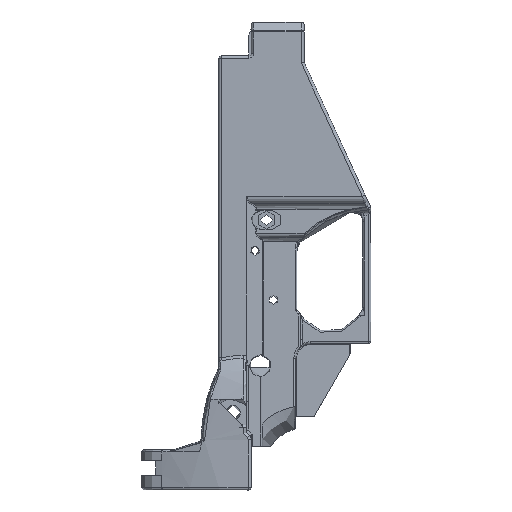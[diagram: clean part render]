
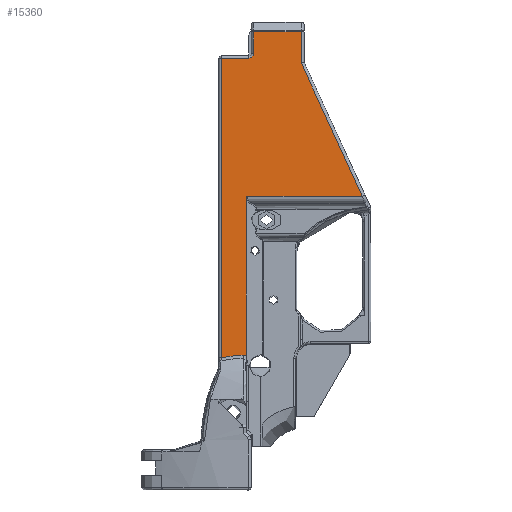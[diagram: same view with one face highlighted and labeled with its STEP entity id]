
A CAD part, left-side view. The second image highlights one B-rep face of the part: STEP entity #15360.
In plain terms, the highlighted planar face has unit normal (-1, 0, 0).
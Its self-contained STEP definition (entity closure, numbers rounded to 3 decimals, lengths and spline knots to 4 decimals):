
#220=ELLIPSE('',#16770,1.9201,1.636);
#401=PLANE('',#16768);
#1354=FACE_OUTER_BOUND('',#2313,.T.);
#2313=EDGE_LOOP('',(#12291,#12292,#12293,#12294,#12295,#12296,#12297,#12298,
#12299,#12300,#12301,#12302));
#3210=B_SPLINE_CURVE_WITH_KNOTS('',3,(#42839,#42840,#42841,#42842),
 .UNSPECIFIED.,.F.,.F.,(4,4),(-0.1434,0.),
 .UNSPECIFIED.);
#3211=B_SPLINE_CURVE_WITH_KNOTS('',3,(#42846,#42847,#42848,#42849,#42850,
#42851,#42852,#42853,#42854,#42855,#42856,#42857),.UNSPECIFIED.,.F.,.F.,
(4,2,2,2,2,4),(-0.117,-0.1147,-0.0798,
-0.057,-0.0072,0.),.UNSPECIFIED.);
#3868=CIRCLE('',#16769,0.08);
#4501=LINE('',#25491,#5269);
#4503=LINE('',#25522,#5271);
#4684=LINE('',#42791,#5452);
#4688=LINE('',#42829,#5456);
#4689=LINE('',#42833,#5457);
#4690=LINE('',#42835,#5458);
#4691=LINE('',#42844,#5459);
#4692=LINE('',#42858,#5460);
#5269=VECTOR('',#18975,0.3937);
#5271=VECTOR('',#18987,0.3937);
#5452=VECTOR('',#19842,0.3937);
#5456=VECTOR('',#19864,0.3937);
#5457=VECTOR('',#19867,0.3937);
#5458=VECTOR('',#19868,0.3937);
#5459=VECTOR('',#19871,1.6985);
#5460=VECTOR('',#19872,0.1181);
#6250=VERTEX_POINT('',#25488);
#6251=VERTEX_POINT('',#25490);
#6255=VERTEX_POINT('',#25520);
#6729=VERTEX_POINT('',#42789);
#6734=VERTEX_POINT('',#42828);
#6735=VERTEX_POINT('',#42830);
#6736=VERTEX_POINT('',#42832);
#6737=VERTEX_POINT('',#42834);
#6738=VERTEX_POINT('',#42836);
#6739=VERTEX_POINT('',#42838);
#6740=VERTEX_POINT('',#42843);
#6741=VERTEX_POINT('',#42845);
#7998=EDGE_CURVE('',#6250,#6251,#4501,.T.);
#8005=EDGE_CURVE('',#6255,#6250,#4503,.T.);
#8711=EDGE_CURVE('',#6729,#6255,#4684,.T.);
#8720=EDGE_CURVE('',#6734,#6729,#4688,.T.);
#8721=EDGE_CURVE('',#6735,#6734,#3868,.T.);
#8722=EDGE_CURVE('',#6736,#6735,#4689,.T.);
#8723=EDGE_CURVE('',#6737,#6736,#4690,.T.);
#8724=EDGE_CURVE('',#6738,#6737,#220,.T.);
#8725=EDGE_CURVE('',#6739,#6738,#3210,.T.);
#8726=EDGE_CURVE('',#6740,#6739,#4691,.T.);
#8727=EDGE_CURVE('',#6741,#6740,#3211,.T.);
#8728=EDGE_CURVE('',#6251,#6741,#4692,.T.);
#12291=ORIENTED_EDGE('',*,*,#7998,.F.);
#12292=ORIENTED_EDGE('',*,*,#8005,.F.);
#12293=ORIENTED_EDGE('',*,*,#8711,.F.);
#12294=ORIENTED_EDGE('',*,*,#8720,.F.);
#12295=ORIENTED_EDGE('',*,*,#8721,.F.);
#12296=ORIENTED_EDGE('',*,*,#8722,.F.);
#12297=ORIENTED_EDGE('',*,*,#8723,.F.);
#12298=ORIENTED_EDGE('',*,*,#8724,.F.);
#12299=ORIENTED_EDGE('',*,*,#8725,.F.);
#12300=ORIENTED_EDGE('',*,*,#8726,.F.);
#12301=ORIENTED_EDGE('',*,*,#8727,.F.);
#12302=ORIENTED_EDGE('',*,*,#8728,.F.);
#15360=ADVANCED_FACE('',(#1354),#401,.F.);
#16768=AXIS2_PLACEMENT_3D('',#42827,#19862,#19863);
#16769=AXIS2_PLACEMENT_3D('',#42831,#19865,#19866);
#16770=AXIS2_PLACEMENT_3D('',#42837,#19869,#19870);
#18975=DIRECTION('',(0.,-0.417,-0.909));
#18987=DIRECTION('',(0.,0.,-1.));
#19842=DIRECTION('',(0.,-1.,0.));
#19862=DIRECTION('center_axis',(1.,0.,0.));
#19863=DIRECTION('ref_axis',(0.,0.,
-1.));
#19864=DIRECTION('',(0.,0.,1.));
#19865=DIRECTION('center_axis',(-1.,0.,0.));
#19866=DIRECTION('ref_axis',(0.,-0.707,-0.707));
#19867=DIRECTION('',(0.,-1.,0.));
#19868=DIRECTION('',(0.,0.,1.));
#19869=DIRECTION('center_axis',(-1.,0.,0.));
#19870=DIRECTION('ref_axis',(0.,-0.984,-0.179));
#19871=DIRECTION('',(0.,0.,-1.));
#19872=DIRECTION('',(0.,1.,0.));
#25488=CARTESIAN_POINT('',(-0.731,-0.0727,2.8507));
#25490=CARTESIAN_POINT('',(-0.731,-1.118,0.5717));
#25491=CARTESIAN_POINT('',(-0.731,-1.4648,-0.1846));
#25520=CARTESIAN_POINT('',(-0.731,-0.0728,3.3816));
#25522=CARTESIAN_POINT('',(-0.731,-0.0727,-0.2092));
#42789=CARTESIAN_POINT('',(-0.731,0.7372,3.3816));
#42791=CARTESIAN_POINT('',(-0.731,0.7121,3.3816));
#42827=CARTESIAN_POINT('Origin',(-0.731,0.68,-3.6849));
#42828=CARTESIAN_POINT('',(-0.731,0.7373,3.0095));
#42829=CARTESIAN_POINT('',(-0.731,0.7373,-0.0118));
#42830=CARTESIAN_POINT('',(-0.731,0.8173,2.9295));
#42831=CARTESIAN_POINT('Origin',(-0.731,0.8173,3.0095));
#42832=CARTESIAN_POINT('',(-0.731,1.2902,2.9295));
#42833=CARTESIAN_POINT('',(-0.731,0.7441,2.9295));
#42834=CARTESIAN_POINT('',(-0.731,1.2902,-2.1813));
#42835=CARTESIAN_POINT('',(-0.731,1.2902,-3.1756));
#42836=CARTESIAN_POINT('',(-0.731,0.9158,-2.1342));
#42837=CARTESIAN_POINT('Origin',(-0.731,0.7244,-3.7785));
#42838=CARTESIAN_POINT('',(-0.731,0.8628,-2.151));
#42839=CARTESIAN_POINT('Ctrl Pts',(-0.731,0.8629,
-2.151));
#42840=CARTESIAN_POINT('Ctrl Pts',(-0.731,0.8784,
-2.1404));
#42841=CARTESIAN_POINT('Ctrl Pts',(-0.731,0.8969,
-2.1335));
#42842=CARTESIAN_POINT('Ctrl Pts',(-0.731,0.9158,
-2.1342));
#42843=CARTESIAN_POINT('',(-0.731,0.8628,0.5319));
#42844=CARTESIAN_POINT('',(-0.731,0.8628,-2.5001));
#42845=CARTESIAN_POINT('',(-0.731,0.8546,0.5717));
#42846=CARTESIAN_POINT('Ctrl Pts',(-0.731,0.8546,
0.5717));
#42847=CARTESIAN_POINT('Ctrl Pts',(-0.731,0.8546,
0.5716));
#42848=CARTESIAN_POINT('Ctrl Pts',(-0.731,0.8546,
0.5716));
#42849=CARTESIAN_POINT('Ctrl Pts',(-0.731,0.855,
0.5706));
#42850=CARTESIAN_POINT('Ctrl Pts',(-0.731,0.8564,
0.5674));
#42851=CARTESIAN_POINT('Ctrl Pts',(-0.731,0.8587,
0.5601));
#42852=CARTESIAN_POINT('Ctrl Pts',(-0.731,0.8595,
0.5572));
#42853=CARTESIAN_POINT('Ctrl Pts',(-0.731,0.8617,
0.5478));
#42854=CARTESIAN_POINT('Ctrl Pts',(-0.731,0.8626,
0.5413));
#42855=CARTESIAN_POINT('Ctrl Pts',(-0.731,0.8628,
0.5338));
#42856=CARTESIAN_POINT('Ctrl Pts',(-0.731,0.8628,
0.5329));
#42857=CARTESIAN_POINT('Ctrl Pts',(-0.731,0.8628,
0.5319));
#42858=CARTESIAN_POINT('',(-0.731,1.0895,0.5717));
